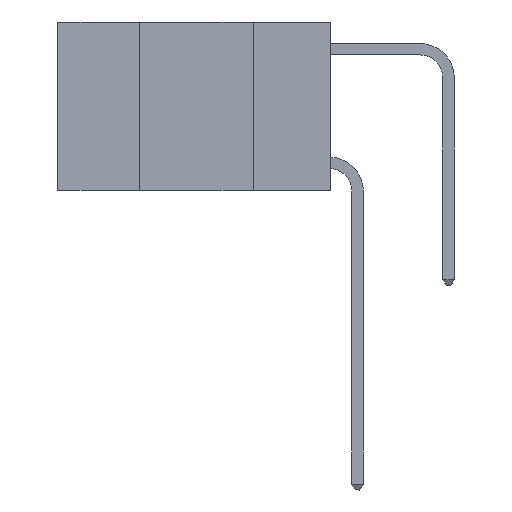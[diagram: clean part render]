
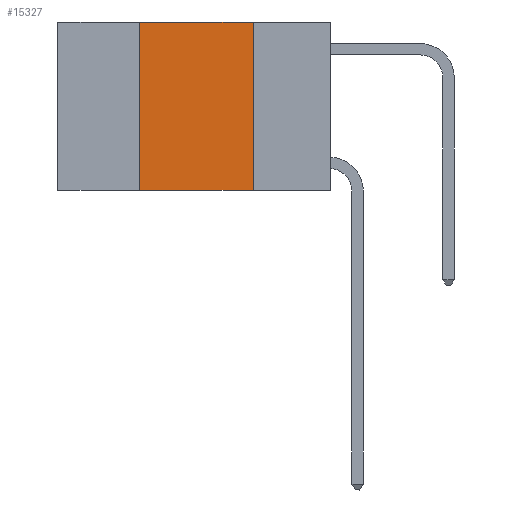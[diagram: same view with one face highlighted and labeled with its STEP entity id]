
A CAD part, left-side view. The second image highlights one B-rep face of the part: STEP entity #15327.
In plain terms, the highlighted planar face has unit normal (-1, 0, 0).
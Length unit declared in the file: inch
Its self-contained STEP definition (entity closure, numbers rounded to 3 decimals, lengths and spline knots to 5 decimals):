
#443 = CARTESIAN_POINT ( 'NONE',  ( 0., 0.42, 0. ) ) ;
#749 = DIRECTION ( 'NONE',  ( 0., 0., -1. ) ) ;
#1510 = DIRECTION ( 'NONE',  ( 0., 0., -1. ) ) ;
#1993 = VERTEX_POINT ( 'NONE', #4607 ) ;
#2178 = EDGE_LOOP ( 'NONE', ( #22996, #7763, #19004, #3636 ) ) ;
#2972 = EDGE_CURVE ( 'NONE', #25532, #8912, #22758, .T. ) ;
#3636 = ORIENTED_EDGE ( 'NONE', *, *, #7026, .T. ) ;
#4607 = CARTESIAN_POINT ( 'NONE',  ( 0., 0.17, -0.37 ) ) ;
#4958 = CARTESIAN_POINT ( 'NONE',  ( 0., 0.42, -0.37 ) ) ;
#5467 = CARTESIAN_POINT ( 'NONE',  ( 0., 0.6, -0.37 ) ) ;
#6853 = LINE ( 'NONE', #12751, #22099 ) ;
#7026 = EDGE_CURVE ( 'NONE', #25532, #1993, #17382, .T. ) ;
#7624 = VECTOR ( 'NONE', #1510, 39.37008 ) ;
#7744 = EDGE_CURVE ( 'NONE', #18238, #1993, #23469, .T. ) ;
#7763 = ORIENTED_EDGE ( 'NONE', *, *, #25397, .F. ) ;
#8912 = VERTEX_POINT ( 'NONE', #443 ) ;
#10898 = PLANE ( 'NONE',  #19920 ) ;
#11478 = VECTOR ( 'NONE', #11507, 39.37008 ) ;
#11507 = DIRECTION ( 'NONE',  ( 0., -1., 0. ) ) ;
#12267 = CARTESIAN_POINT ( 'NONE',  ( 0., 0.17, 0. ) ) ;
#12751 = CARTESIAN_POINT ( 'NONE',  ( 0., 0.6, 0. ) ) ;
#12891 = DIRECTION ( 'NONE',  ( 1., 0., 0. ) ) ;
#14732 = DIRECTION ( 'NONE',  ( 0., -1., 0. ) ) ;
#15282 = FACE_OUTER_BOUND ( 'NONE', #2178, .T. ) ;
#15327 = ADVANCED_FACE ( 'NONE', ( #15282 ), #10898, .F. ) ;
#15370 = DIRECTION ( 'NONE',  ( 0., 0., 1. ) ) ;
#17382 = LINE ( 'NONE', #5467, #11478 ) ;
#18238 = VERTEX_POINT ( 'NONE', #12267 ) ;
#19004 = ORIENTED_EDGE ( 'NONE', *, *, #2972, .F. ) ;
#19576 = CARTESIAN_POINT ( 'NONE',  ( 0., 0.17, 0. ) ) ;
#19920 = AXIS2_PLACEMENT_3D ( 'NONE', #24674, #12891, #749 ) ;
#21524 = VECTOR ( 'NONE', #15370, 39.37008 ) ;
#22099 = VECTOR ( 'NONE', #14732, 39.37008 ) ;
#22758 = LINE ( 'NONE', #24831, #21524 ) ;
#22996 = ORIENTED_EDGE ( 'NONE', *, *, #7744, .F. ) ;
#23469 = LINE ( 'NONE', #19576, #7624 ) ;
#24674 = CARTESIAN_POINT ( 'NONE',  ( 0., 0.6, 0. ) ) ;
#24831 = CARTESIAN_POINT ( 'NONE',  ( 0., 0.42, 0. ) ) ;
#25397 = EDGE_CURVE ( 'NONE', #8912, #18238, #6853, .T. ) ;
#25532 = VERTEX_POINT ( 'NONE', #4958 ) ;
